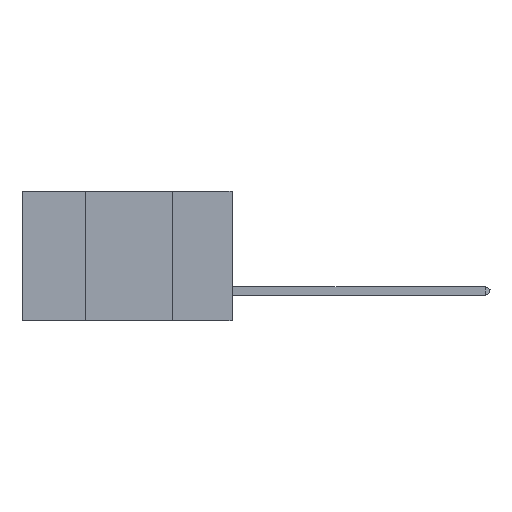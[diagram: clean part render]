
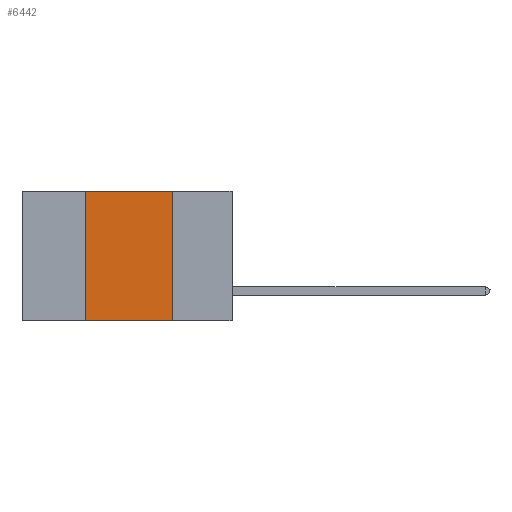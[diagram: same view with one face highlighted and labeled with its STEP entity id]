
A CAD part, left-side view. The second image highlights one B-rep face of the part: STEP entity #6442.
In plain terms, the highlighted planar face has unit normal (-1, 0, 0).
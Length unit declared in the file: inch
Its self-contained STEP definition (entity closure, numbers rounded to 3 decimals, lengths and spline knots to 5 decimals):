
#140 = CARTESIAN_POINT ( 'NONE',  ( 0., 0.42, 0. ) ) ;
#234 = ORIENTED_EDGE ( 'NONE', *, *, #291, .F. ) ;
#291 = EDGE_CURVE ( 'NONE', #9467, #12599, #2344, .T. ) ;
#1156 = FACE_OUTER_BOUND ( 'NONE', #8819, .T. ) ;
#1651 = VECTOR ( 'NONE', #6366, 39.37008 ) ;
#1747 = CARTESIAN_POINT ( 'NONE',  ( 0., 0.6, 0. ) ) ;
#1765 = DIRECTION ( 'NONE',  ( 0., -1., 0. ) ) ;
#1772 = LINE ( 'NONE', #8642, #14648 ) ;
#1941 = CARTESIAN_POINT ( 'NONE',  ( 0., 0.42, 0. ) ) ;
#1979 = CARTESIAN_POINT ( 'NONE',  ( 0., 0.17, 0. ) ) ;
#2295 = CARTESIAN_POINT ( 'NONE',  ( 0., 0.6, 0. ) ) ;
#2344 = LINE ( 'NONE', #5261, #10375 ) ;
#3065 = CARTESIAN_POINT ( 'NONE',  ( 0., 0.17, -0.37 ) ) ;
#5215 = DIRECTION ( 'NONE',  ( 0., 0., -1. ) ) ;
#5261 = CARTESIAN_POINT ( 'NONE',  ( 0., 0.17, 0. ) ) ;
#5534 = DIRECTION ( 'NONE',  ( 0., 0., -1. ) ) ;
#6366 = DIRECTION ( 'NONE',  ( 0., -1., 0. ) ) ;
#6442 = ADVANCED_FACE ( 'NONE', ( #1156 ), #10184, .F. ) ;
#6774 = DIRECTION ( 'NONE',  ( 1., 0., 0. ) ) ;
#7225 = AXIS2_PLACEMENT_3D ( 'NONE', #2295, #6774, #5534 ) ;
#7995 = EDGE_CURVE ( 'NONE', #12271, #9467, #14186, .T. ) ;
#8219 = LINE ( 'NONE', #1941, #14457 ) ;
#8642 = CARTESIAN_POINT ( 'NONE',  ( 0., 0.6, -0.37 ) ) ;
#8819 = EDGE_LOOP ( 'NONE', ( #234, #9792, #8902, #9372 ) ) ;
#8902 = ORIENTED_EDGE ( 'NONE', *, *, #10771, .F. ) ;
#9372 = ORIENTED_EDGE ( 'NONE', *, *, #9937, .T. ) ;
#9467 = VERTEX_POINT ( 'NONE', #1979 ) ;
#9792 = ORIENTED_EDGE ( 'NONE', *, *, #7995, .F. ) ;
#9937 = EDGE_CURVE ( 'NONE', #14399, #12599, #1772, .T. ) ;
#10184 = PLANE ( 'NONE',  #7225 ) ;
#10375 = VECTOR ( 'NONE', #5215, 39.37008 ) ;
#10771 = EDGE_CURVE ( 'NONE', #14399, #12271, #8219, .T. ) ;
#11008 = DIRECTION ( 'NONE',  ( 0., 0., 1. ) ) ;
#12168 = CARTESIAN_POINT ( 'NONE',  ( 0., 0.42, -0.37 ) ) ;
#12271 = VERTEX_POINT ( 'NONE', #140 ) ;
#12599 = VERTEX_POINT ( 'NONE', #3065 ) ;
#14186 = LINE ( 'NONE', #1747, #1651 ) ;
#14399 = VERTEX_POINT ( 'NONE', #12168 ) ;
#14457 = VECTOR ( 'NONE', #11008, 39.37008 ) ;
#14648 = VECTOR ( 'NONE', #1765, 39.37008 ) ;
